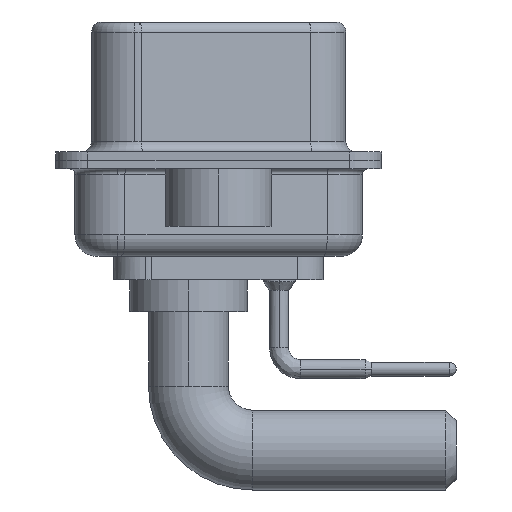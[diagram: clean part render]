
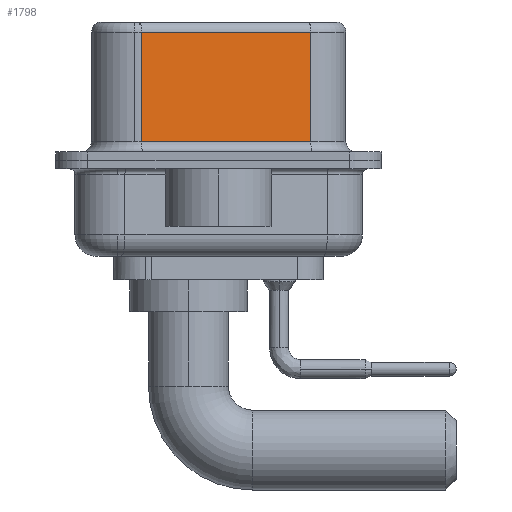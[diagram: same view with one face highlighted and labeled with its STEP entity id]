
A CAD part, left-side view. The second image highlights one B-rep face of the part: STEP entity #1798.
In plain terms, the highlighted planar face has unit normal (-0.985, -0.174, 0).
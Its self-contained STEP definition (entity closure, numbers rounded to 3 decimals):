
#434 = DIRECTION ( 'NONE',  ( -0.174, 0.985, 0. ) ) ;
#1647 = CARTESIAN_POINT ( 'NONE',  ( 3.73, 3.628, 6.52 ) ) ;
#1798 = ADVANCED_FACE ( 'NONE', ( #5123 ), #10911, .F. ) ;
#2734 = CARTESIAN_POINT ( 'NONE',  ( 3.73, 3.628, 0.9 ) ) ;
#2965 = VECTOR ( 'NONE', #13805, 1000. ) ;
#3292 = DIRECTION ( 'NONE',  ( 0.985, 0.174, 0. ) ) ;
#3451 = CARTESIAN_POINT ( 'NONE',  ( 5.132, -4.322, 0.9 ) ) ;
#3457 = ORIENTED_EDGE ( 'NONE', *, *, #7659, .T. ) ;
#4131 = ORIENTED_EDGE ( 'NONE', *, *, #18669, .T. ) ;
#5123 = FACE_OUTER_BOUND ( 'NONE', #16173, .T. ) ;
#5633 = LINE ( 'NONE', #1647, #14619 ) ;
#7659 = EDGE_CURVE ( 'NONE', #16254, #8732, #18947, .T. ) ;
#7827 = VERTEX_POINT ( 'NONE', #2734 ) ;
#8058 = EDGE_CURVE ( 'NONE', #16254, #12246, #17183, .T. ) ;
#8182 = CARTESIAN_POINT ( 'NONE',  ( 5.132, -4.322, 6.02 ) ) ;
#8732 = VERTEX_POINT ( 'NONE', #21863 ) ;
#9346 = EDGE_CURVE ( 'NONE', #7827, #12246, #10837, .T. ) ;
#9374 = ORIENTED_EDGE ( 'NONE', *, *, #9346, .T. ) ;
#9799 = CARTESIAN_POINT ( 'NONE',  ( 5.132, -4.322, 6.52 ) ) ;
#10675 = DIRECTION ( 'NONE',  ( -0.174, 0.985, 0. ) ) ;
#10837 = LINE ( 'NONE', #3451, #18330 ) ;
#10911 = PLANE ( 'NONE',  #20699 ) ;
#12246 = VERTEX_POINT ( 'NONE', #15984 ) ;
#13805 = DIRECTION ( 'NONE',  ( 0., 0., -1. ) ) ;
#14619 = VECTOR ( 'NONE', #16515, 1000. ) ;
#14922 = DIRECTION ( 'NONE',  ( 0.174, -0.985, 0. ) ) ;
#15984 = CARTESIAN_POINT ( 'NONE',  ( 5.132, -4.322, 0.9 ) ) ;
#16173 = EDGE_LOOP ( 'NONE', ( #19556, #3457, #4131, #9374 ) ) ;
#16254 = VERTEX_POINT ( 'NONE', #19543 ) ;
#16515 = DIRECTION ( 'NONE',  ( 0., 0., -1. ) ) ;
#17183 = LINE ( 'NONE', #9799, #2965 ) ;
#18330 = VECTOR ( 'NONE', #14922, 1000. ) ;
#18669 = EDGE_CURVE ( 'NONE', #8732, #7827, #5633, .T. ) ;
#18947 = LINE ( 'NONE', #8182, #19955 ) ;
#19543 = CARTESIAN_POINT ( 'NONE',  ( 5.132, -4.322, 6.02 ) ) ;
#19556 = ORIENTED_EDGE ( 'NONE', *, *, #8058, .F. ) ;
#19866 = CARTESIAN_POINT ( 'NONE',  ( 5.132, -4.322, 6.52 ) ) ;
#19955 = VECTOR ( 'NONE', #434, 1000. ) ;
#20699 = AXIS2_PLACEMENT_3D ( 'NONE', #19866, #3292, #10675 ) ;
#21863 = CARTESIAN_POINT ( 'NONE',  ( 3.73, 3.628, 6.02 ) ) ;
